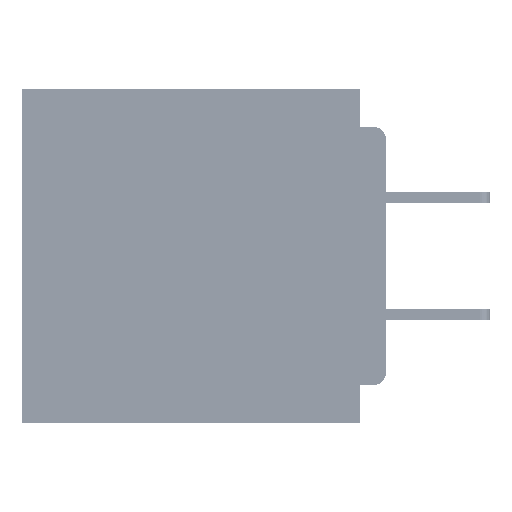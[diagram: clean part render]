
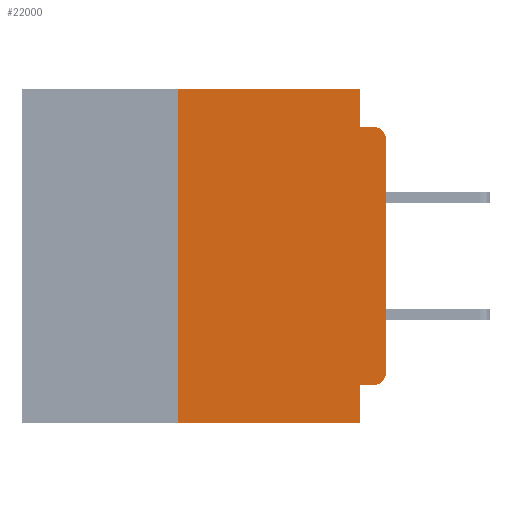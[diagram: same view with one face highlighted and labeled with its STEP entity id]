
A CAD part, left-side view. The second image highlights one B-rep face of the part: STEP entity #22000.
In plain terms, the highlighted planar face has unit normal (-1, 0, 0).
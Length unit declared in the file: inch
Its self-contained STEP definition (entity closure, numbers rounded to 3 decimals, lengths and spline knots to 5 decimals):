
#1432 = DIRECTION ( 'NONE',  ( 0., 0., 1. ) ) ;
#1575 = EDGE_CURVE ( 'NONE', #31962, #17001, #17791, .T. ) ;
#1900 = DIRECTION ( 'NONE',  ( -1., 0., 0. ) ) ;
#3315 = EDGE_CURVE ( 'NONE', #20152, #23579, #30392, .T. ) ;
#4817 = VERTEX_POINT ( 'NONE', #18984 ) ;
#5826 = EDGE_CURVE ( 'NONE', #26497, #65630, #58583, .T. ) ;
#7144 = CARTESIAN_POINT ( 'NONE',  ( 0., 0.437, -0.4 ) ) ;
#7876 = VECTOR ( 'NONE', #27728, 39.37008 ) ;
#9335 = DIRECTION ( 'NONE',  ( 1., 0., 0. ) ) ;
#15162 = ORIENTED_EDGE ( 'NONE', *, *, #59347, .T. ) ;
#15253 = VECTOR ( 'NONE', #28212, 39.37008 ) ;
#15415 = EDGE_CURVE ( 'NONE', #47361, #26497, #65579, .T. ) ;
#16352 = CARTESIAN_POINT ( 'NONE',  ( 0., 0.031, -0.4 ) ) ;
#16591 = DIRECTION ( 'NONE',  ( -1., 0., 0. ) ) ;
#16689 = CARTESIAN_POINT ( 'NONE',  ( 0., 0., 0. ) ) ;
#17001 = VERTEX_POINT ( 'NONE', #25781 ) ;
#17791 = LINE ( 'NONE', #56454, #59411 ) ;
#18897 = CARTESIAN_POINT ( 'NONE',  ( 0., 0.437, 0. ) ) ;
#18984 = CARTESIAN_POINT ( 'NONE',  ( 0., 0.031, 0. ) ) ;
#19128 = EDGE_CURVE ( 'NONE', #50102, #23579, #42247, .T. ) ;
#19281 = EDGE_CURVE ( 'NONE', #31962, #65630, #20901, .T. ) ;
#20152 = VERTEX_POINT ( 'NONE', #52109 ) ;
#20901 = LINE ( 'NONE', #7144, #62508 ) ;
#22000 = ADVANCED_FACE ( 'NONE', ( #26498 ), #41925, .F. ) ;
#22641 = CARTESIAN_POINT ( 'NONE',  ( 0., 0.031, -0.4 ) ) ;
#22814 = VECTOR ( 'NONE', #67720, 39.37008 ) ;
#23579 = VERTEX_POINT ( 'NONE', #56260 ) ;
#25781 = CARTESIAN_POINT ( 'NONE',  ( 0., 0.25, 0. ) ) ;
#25905 = CARTESIAN_POINT ( 'NONE',  ( 0., 0.031, -0.355 ) ) ;
#26497 = VERTEX_POINT ( 'NONE', #25905 ) ;
#26498 = FACE_OUTER_BOUND ( 'NONE', #47909, .T. ) ;
#27651 = AXIS2_PLACEMENT_3D ( 'NONE', #63419, #9335, #47379 ) ;
#27710 = CARTESIAN_POINT ( 'NONE',  ( 0., 0., -0.045 ) ) ;
#27728 = DIRECTION ( 'NONE',  ( 0., 1., 0. ) ) ;
#27830 = VECTOR ( 'NONE', #33168, 39.37008 ) ;
#28212 = DIRECTION ( 'NONE',  ( 0., 0., -1. ) ) ;
#28794 = ORIENTED_EDGE ( 'NONE', *, *, #54120, .T. ) ;
#29077 = DIRECTION ( 'NONE',  ( 0., 0., -1. ) ) ;
#30392 = CIRCLE ( 'NONE', #57652, 0.015 ) ;
#31962 = VERTEX_POINT ( 'NONE', #60257 ) ;
#33168 = DIRECTION ( 'NONE',  ( 0., -1., 0. ) ) ;
#33554 = ORIENTED_EDGE ( 'NONE', *, *, #5826, .F. ) ;
#34103 = CARTESIAN_POINT ( 'NONE',  ( 0., 0.031, -0.045 ) ) ;
#34451 = CARTESIAN_POINT ( 'NONE',  ( 0., 0., -0.34 ) ) ;
#34582 = CARTESIAN_POINT ( 'NONE',  ( 0., 0.015, -0.06 ) ) ;
#34701 = DIRECTION ( 'NONE',  ( 0., 0., 1. ) ) ;
#34793 = CIRCLE ( 'NONE', #38994, 0.015 ) ;
#35623 = EDGE_CURVE ( 'NONE', #4817, #50102, #68176, .T. ) ;
#35816 = ORIENTED_EDGE ( 'NONE', *, *, #15415, .F. ) ;
#38389 = CARTESIAN_POINT ( 'NONE',  ( 0., 0., -0.355 ) ) ;
#38704 = ORIENTED_EDGE ( 'NONE', *, *, #35623, .F. ) ;
#38799 = ORIENTED_EDGE ( 'NONE', *, *, #67001, .F. ) ;
#38994 = AXIS2_PLACEMENT_3D ( 'NONE', #49175, #16591, #54567 ) ;
#39700 = ORIENTED_EDGE ( 'NONE', *, *, #1575, .F. ) ;
#40023 = DIRECTION ( 'NONE',  ( 0., 0., -1. ) ) ;
#41925 = PLANE ( 'NONE',  #27651 ) ;
#42247 = LINE ( 'NONE', #27710, #27830 ) ;
#43022 = CARTESIAN_POINT ( 'NONE',  ( 0., 0.015, -0.355 ) ) ;
#47361 = VERTEX_POINT ( 'NONE', #43022 ) ;
#47379 = DIRECTION ( 'NONE',  ( 0., 0., -1. ) ) ;
#47909 = EDGE_LOOP ( 'NONE', ( #28794, #63552, #55900, #38704, #38799, #39700, #54625, #33554, #35816, #15162 ) ) ;
#49175 = CARTESIAN_POINT ( 'NONE',  ( 0., 0.015, -0.34 ) ) ;
#50102 = VERTEX_POINT ( 'NONE', #34103 ) ;
#50679 = DIRECTION ( 'NONE',  ( 0., -1., 0. ) ) ;
#52109 = CARTESIAN_POINT ( 'NONE',  ( 0., 0., -0.06 ) ) ;
#54120 = EDGE_CURVE ( 'NONE', #61564, #20152, #56632, .T. ) ;
#54567 = DIRECTION ( 'NONE',  ( 0., 0., -1. ) ) ;
#54625 = ORIENTED_EDGE ( 'NONE', *, *, #19281, .T. ) ;
#55900 = ORIENTED_EDGE ( 'NONE', *, *, #19128, .F. ) ;
#56260 = CARTESIAN_POINT ( 'NONE',  ( 0., 0.015, -0.045 ) ) ;
#56454 = CARTESIAN_POINT ( 'NONE',  ( 0., 0.25, -0.4 ) ) ;
#56632 = LINE ( 'NONE', #16689, #69240 ) ;
#57652 = AXIS2_PLACEMENT_3D ( 'NONE', #34582, #1900, #40023 ) ;
#58583 = LINE ( 'NONE', #22641, #15253 ) ;
#59347 = EDGE_CURVE ( 'NONE', #47361, #61564, #34793, .T. ) ;
#59411 = VECTOR ( 'NONE', #34701, 39.37008 ) ;
#60257 = CARTESIAN_POINT ( 'NONE',  ( 0., 0.25, -0.4 ) ) ;
#61564 = VERTEX_POINT ( 'NONE', #34451 ) ;
#62508 = VECTOR ( 'NONE', #50679, 39.37008 ) ;
#63150 = VECTOR ( 'NONE', #29077, 39.37008 ) ;
#63419 = CARTESIAN_POINT ( 'NONE',  ( 0., 0.437, 0. ) ) ;
#63552 = ORIENTED_EDGE ( 'NONE', *, *, #3315, .T. ) ;
#65006 = CARTESIAN_POINT ( 'NONE',  ( 0., 0.031, 0. ) ) ;
#65579 = LINE ( 'NONE', #38389, #7876 ) ;
#65630 = VERTEX_POINT ( 'NONE', #16352 ) ;
#67001 = EDGE_CURVE ( 'NONE', #17001, #4817, #67765, .T. ) ;
#67720 = DIRECTION ( 'NONE',  ( 0., -1., 0. ) ) ;
#67765 = LINE ( 'NONE', #18897, #22814 ) ;
#68176 = LINE ( 'NONE', #65006, #63150 ) ;
#69240 = VECTOR ( 'NONE', #1432, 39.37008 ) ;
